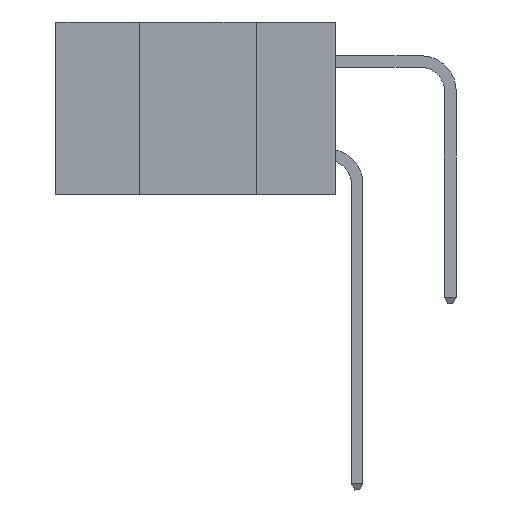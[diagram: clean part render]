
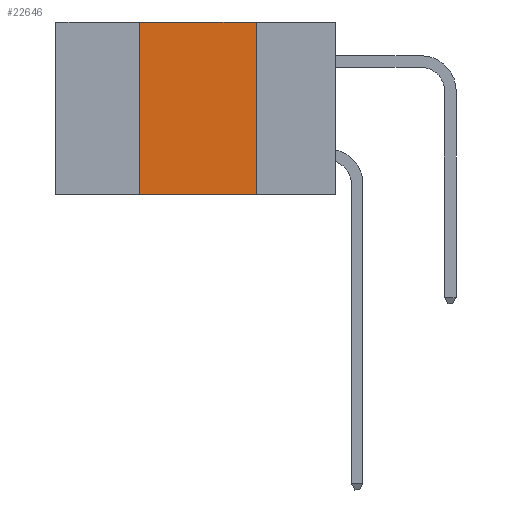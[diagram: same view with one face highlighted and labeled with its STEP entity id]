
A CAD part, left-side view. The second image highlights one B-rep face of the part: STEP entity #22646.
In plain terms, the highlighted planar face has unit normal (-1, 0, 0).
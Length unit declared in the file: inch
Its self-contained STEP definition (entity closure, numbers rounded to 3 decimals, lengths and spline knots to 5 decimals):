
#269 = FACE_OUTER_BOUND ( 'NONE', #6911, .T. ) ;
#322 = LINE ( 'NONE', #16623, #16317 ) ;
#338 = PLANE ( 'NONE',  #1271 ) ;
#1267 = EDGE_CURVE ( 'NONE', #25545, #19903, #27635, .T. ) ;
#1271 = AXIS2_PLACEMENT_3D ( 'NONE', #26622, #24038, #13423 ) ;
#3754 = VECTOR ( 'NONE', #19610, 39.37008 ) ;
#6675 = VERTEX_POINT ( 'NONE', #21122 ) ;
#6911 = EDGE_LOOP ( 'NONE', ( #33405, #25472, #26170, #27119 ) ) ;
#8809 = DIRECTION ( 'NONE',  ( 0., -1., 0. ) ) ;
#9663 = LINE ( 'NONE', #30207, #3754 ) ;
#10325 = VERTEX_POINT ( 'NONE', #27462 ) ;
#10503 = CARTESIAN_POINT ( 'NONE',  ( 0., 0.6, -0.37 ) ) ;
#11717 = VECTOR ( 'NONE', #14915, 39.37008 ) ;
#13423 = DIRECTION ( 'NONE',  ( 0., 0., -1. ) ) ;
#14915 = DIRECTION ( 'NONE',  ( 0., -1., 0. ) ) ;
#15403 = EDGE_CURVE ( 'NONE', #6675, #10325, #9663, .T. ) ;
#16317 = VECTOR ( 'NONE', #8809, 39.37008 ) ;
#16330 = LINE ( 'NONE', #10503, #11717 ) ;
#16623 = CARTESIAN_POINT ( 'NONE',  ( 0., 0.6, 0. ) ) ;
#17513 = CARTESIAN_POINT ( 'NONE',  ( 0., 0.42, -0.37 ) ) ;
#19610 = DIRECTION ( 'NONE',  ( 0., 0., -1. ) ) ;
#19903 = VERTEX_POINT ( 'NONE', #20200 ) ;
#20200 = CARTESIAN_POINT ( 'NONE',  ( 0., 0.42, 0. ) ) ;
#21122 = CARTESIAN_POINT ( 'NONE',  ( 0., 0.17, 0. ) ) ;
#21998 = EDGE_CURVE ( 'NONE', #25545, #10325, #16330, .T. ) ;
#22459 = DIRECTION ( 'NONE',  ( 0., 0., 1. ) ) ;
#22646 = ADVANCED_FACE ( 'NONE', ( #269 ), #338, .F. ) ;
#24038 = DIRECTION ( 'NONE',  ( 1., 0., 0. ) ) ;
#25472 = ORIENTED_EDGE ( 'NONE', *, *, #29887, .F. ) ;
#25545 = VERTEX_POINT ( 'NONE', #17513 ) ;
#26170 = ORIENTED_EDGE ( 'NONE', *, *, #1267, .F. ) ;
#26622 = CARTESIAN_POINT ( 'NONE',  ( 0., 0.6, 0. ) ) ;
#27119 = ORIENTED_EDGE ( 'NONE', *, *, #21998, .T. ) ;
#27462 = CARTESIAN_POINT ( 'NONE',  ( 0., 0.17, -0.37 ) ) ;
#27635 = LINE ( 'NONE', #30858, #31858 ) ;
#29887 = EDGE_CURVE ( 'NONE', #19903, #6675, #322, .T. ) ;
#30207 = CARTESIAN_POINT ( 'NONE',  ( 0., 0.17, 0. ) ) ;
#30858 = CARTESIAN_POINT ( 'NONE',  ( 0., 0.42, 0. ) ) ;
#31858 = VECTOR ( 'NONE', #22459, 39.37008 ) ;
#33405 = ORIENTED_EDGE ( 'NONE', *, *, #15403, .F. ) ;
